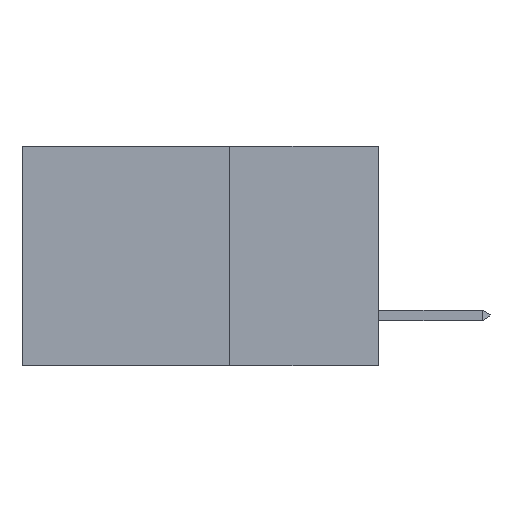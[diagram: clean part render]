
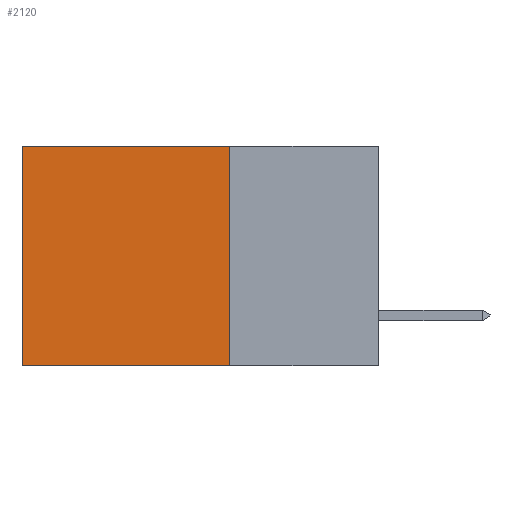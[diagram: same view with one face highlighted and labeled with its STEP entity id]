
A CAD part, left-side view. The second image highlights one B-rep face of the part: STEP entity #2120.
In plain terms, the highlighted planar face has unit normal (-1, 0, 0).
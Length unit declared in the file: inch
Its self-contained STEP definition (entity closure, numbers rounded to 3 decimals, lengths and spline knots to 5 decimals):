
#83 = PLANE ( 'NONE',  #1249 ) ;
#682 = ORIENTED_EDGE ( 'NONE', *, *, #6148, .F. ) ;
#1249 = AXIS2_PLACEMENT_3D ( 'NONE', #2867, #2178, #3037 ) ;
#1401 = CARTESIAN_POINT ( 'NONE',  ( 0.2615, 0.25, -0.37 ) ) ;
#1497 = DIRECTION ( 'NONE',  ( 0., 0., -1. ) ) ;
#1585 = EDGE_CURVE ( 'NONE', #3878, #3872, #6257, .T. ) ;
#1622 = VERTEX_POINT ( 'NONE', #5677 ) ;
#2120 = ADVANCED_FACE ( 'NONE', ( #6300 ), #83, .F. ) ;
#2144 = VECTOR ( 'NONE', #3504, 39.37008 ) ;
#2178 = DIRECTION ( 'NONE',  ( 1., 0., 0. ) ) ;
#2224 = VECTOR ( 'NONE', #6114, 39.37008 ) ;
#2695 = CARTESIAN_POINT ( 'NONE',  ( 0.2615, 0.25, -0.37 ) ) ;
#2867 = CARTESIAN_POINT ( 'NONE',  ( 0.2615, 0.25, -0.37 ) ) ;
#3037 = DIRECTION ( 'NONE',  ( 0., 0., -1. ) ) ;
#3187 = ORIENTED_EDGE ( 'NONE', *, *, #1585, .F. ) ;
#3377 = EDGE_LOOP ( 'NONE', ( #4234, #682, #3187, #7289 ) ) ;
#3504 = DIRECTION ( 'NONE',  ( 0., 1., 0. ) ) ;
#3872 = VERTEX_POINT ( 'NONE', #8244 ) ;
#3878 = VERTEX_POINT ( 'NONE', #4212 ) ;
#4212 = CARTESIAN_POINT ( 'NONE',  ( 0.2615, 0.25, 0. ) ) ;
#4234 = ORIENTED_EDGE ( 'NONE', *, *, #4361, .T. ) ;
#4361 = EDGE_CURVE ( 'NONE', #1622, #7140, #7577, .T. ) ;
#5064 = CARTESIAN_POINT ( 'NONE',  ( 0.2615, 0.25, 0. ) ) ;
#5085 = CARTESIAN_POINT ( 'NONE',  ( 0.2615, 0.6, -0.37 ) ) ;
#5466 = CARTESIAN_POINT ( 'NONE',  ( 0.2615, 0.6, -0.37 ) ) ;
#5541 = VECTOR ( 'NONE', #1497, 39.37008 ) ;
#5677 = CARTESIAN_POINT ( 'NONE',  ( 0.2615, 0.6, 0. ) ) ;
#5906 = EDGE_CURVE ( 'NONE', #3878, #1622, #7215, .T. ) ;
#6114 = DIRECTION ( 'NONE',  ( 0., 0., -1. ) ) ;
#6148 = EDGE_CURVE ( 'NONE', #3872, #7140, #6846, .T. ) ;
#6257 = LINE ( 'NONE', #1401, #5541 ) ;
#6300 = FACE_OUTER_BOUND ( 'NONE', #3377, .T. ) ;
#6846 = LINE ( 'NONE', #2695, #2144 ) ;
#7060 = VECTOR ( 'NONE', #7126, 39.37008 ) ;
#7126 = DIRECTION ( 'NONE',  ( 0., 1., 0. ) ) ;
#7140 = VERTEX_POINT ( 'NONE', #5085 ) ;
#7215 = LINE ( 'NONE', #5064, #7060 ) ;
#7289 = ORIENTED_EDGE ( 'NONE', *, *, #5906, .T. ) ;
#7577 = LINE ( 'NONE', #5466, #2224 ) ;
#8244 = CARTESIAN_POINT ( 'NONE',  ( 0.2615, 0.25, -0.37 ) ) ;
